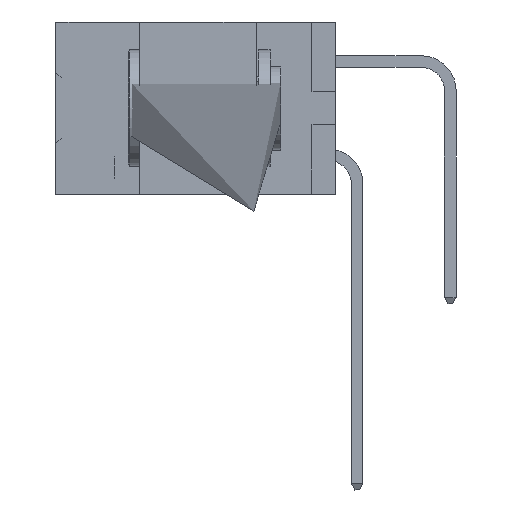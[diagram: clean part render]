
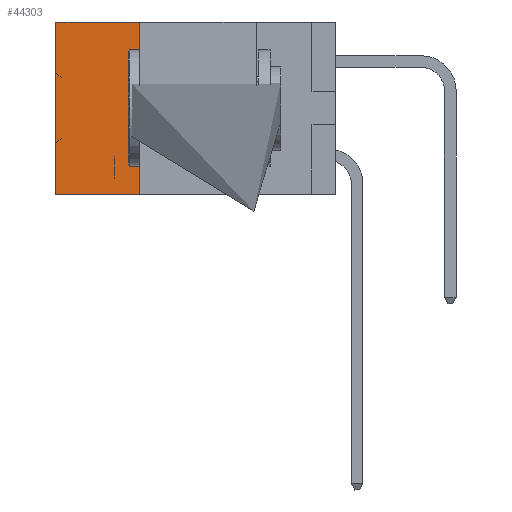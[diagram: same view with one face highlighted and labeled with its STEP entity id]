
A CAD part, left-side view. The second image highlights one B-rep face of the part: STEP entity #44303.
In plain terms, the highlighted planar face has unit normal (-1, 0, 0).
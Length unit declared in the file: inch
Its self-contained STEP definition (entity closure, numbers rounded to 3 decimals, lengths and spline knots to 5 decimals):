
#4600 = VERTEX_POINT ( 'NONE', #9716 ) ;
#5384 = EDGE_CURVE ( 'NONE', #4600, #41570, #47593, .T. ) ;
#6545 = VERTEX_POINT ( 'NONE', #44791 ) ;
#6551 = PLANE ( 'NONE',  #43721 ) ;
#9477 = EDGE_CURVE ( 'NONE', #6545, #12259, #47664, .T. ) ;
#9716 = CARTESIAN_POINT ( 'NONE',  ( 0.2875, 0.42, 0. ) ) ;
#10304 = LINE ( 'NONE', #31871, #42096 ) ;
#12259 = VERTEX_POINT ( 'NONE', #26190 ) ;
#17606 = CARTESIAN_POINT ( 'NONE',  ( 0.2875, 0.42, -0.37 ) ) ;
#19210 = DIRECTION ( 'NONE',  ( 0., 0., -1. ) ) ;
#19967 = VECTOR ( 'NONE', #29739, 39.37008 ) ;
#21614 = VECTOR ( 'NONE', #24057, 39.37008 ) ;
#23235 = LINE ( 'NONE', #17606, #19967 ) ;
#23490 = EDGE_CURVE ( 'NONE', #4600, #6545, #10304, .T. ) ;
#24057 = DIRECTION ( 'NONE',  ( 0., 0., -1. ) ) ;
#24965 = VECTOR ( 'NONE', #37538, 39.37008 ) ;
#26190 = CARTESIAN_POINT ( 'NONE',  ( 0.2875, 0.6, -0.37 ) ) ;
#27355 = CARTESIAN_POINT ( 'NONE',  ( 0.2875, 0.42, 0. ) ) ;
#29739 = DIRECTION ( 'NONE',  ( 0., 1., 0. ) ) ;
#31871 = CARTESIAN_POINT ( 'NONE',  ( 0.2875, 0.42, 0. ) ) ;
#32417 = EDGE_CURVE ( 'NONE', #41570, #12259, #23235, .T. ) ;
#35503 = DIRECTION ( 'NONE',  ( 1., 0., 0. ) ) ;
#36267 = CARTESIAN_POINT ( 'NONE',  ( 0.2875, 0.42, -0.37 ) ) ;
#36938 = CARTESIAN_POINT ( 'NONE',  ( 0.2875, 0.42, 0. ) ) ;
#37538 = DIRECTION ( 'NONE',  ( 0., 0., -1. ) ) ;
#41522 = CARTESIAN_POINT ( 'NONE',  ( 0.2875, 0.6, 0. ) ) ;
#41570 = VERTEX_POINT ( 'NONE', #36267 ) ;
#42096 = VECTOR ( 'NONE', #49987, 39.37008 ) ;
#43140 = ORIENTED_EDGE ( 'NONE', *, *, #5384, .F. ) ;
#43709 = FACE_OUTER_BOUND ( 'NONE', #48232, .T. ) ;
#43721 = AXIS2_PLACEMENT_3D ( 'NONE', #27355, #35503, #19210 ) ;
#44303 = ADVANCED_FACE ( 'NONE', ( #43709 ), #6551, .F. ) ;
#44791 = CARTESIAN_POINT ( 'NONE',  ( 0.2875, 0.6, 0. ) ) ;
#46193 = ORIENTED_EDGE ( 'NONE', *, *, #23490, .T. ) ;
#47593 = LINE ( 'NONE', #36938, #21614 ) ;
#47664 = LINE ( 'NONE', #41522, #24965 ) ;
#47958 = ORIENTED_EDGE ( 'NONE', *, *, #32417, .F. ) ;
#48232 = EDGE_LOOP ( 'NONE', ( #52187, #47958, #43140, #46193 ) ) ;
#49987 = DIRECTION ( 'NONE',  ( 0., 1., 0. ) ) ;
#52187 = ORIENTED_EDGE ( 'NONE', *, *, #9477, .T. ) ;
